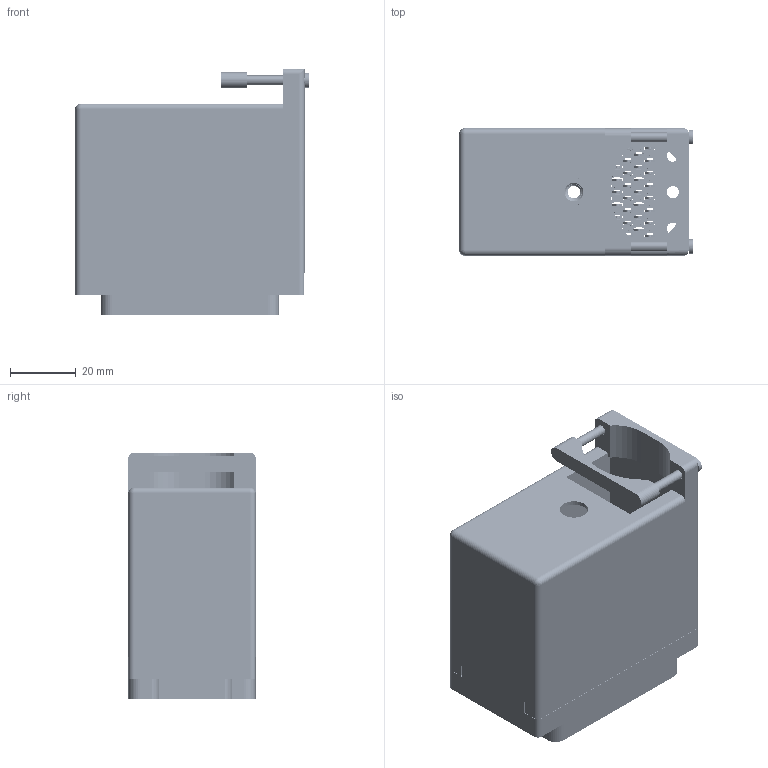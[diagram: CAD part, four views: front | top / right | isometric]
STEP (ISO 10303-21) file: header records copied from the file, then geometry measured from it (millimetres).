
FILE_DESCRIPTION (( 'STEP AP203' ), '1' );
FILE_NAME ('516-120-540-366.STEP', '2020-03-11T05:23:50', ( '' ), ( '' ), 'SwSTEP 2.0', 'SolidWorks 2016', '' );
FILE_SCHEMA (( 'CONFIG_CONTROL_DESIGN' ));
Length unit declared in the file: inch
Products named in the file (5): 516-230-001_Metal - 120 Top Entry; 516-252-095-100; 516-120-540-366; 516 Plug Insulator_120; 516-292-001_540 Contact
Assembly tree (123 placements, depth 2):
  516-120-540-366
    516 Plug Insulator_120
    516-292-001_540 Contact  x120
    516-230-001_Metal - 120 Top Entry
    516-252-095-100
Bounding box: 71.25 x 38.86 x 75.26 mm (x, y, z)
Volume: 43092.1 mm3; surface area: 79645.1 mm2
Topology: 123 solids, 123 shells, 11134 faces, 32363 edges, 21487 vertices
Faces by surface type: plane 6884, cylinder 3510, bspline 726, cone 12, sphere 2
Entity records: 92698 total; most frequent: CARTESIAN_POINT 17693, ORIENTED_EDGE 15218, DIRECTION 14660, EDGE_CURVE 7609, VECTOR 5742, LINE 5742, VERTEX_POINT 5065, AXIS2_PLACEMENT_3D 4459
